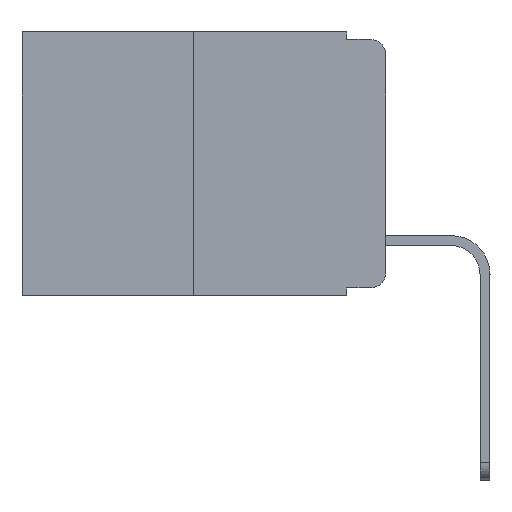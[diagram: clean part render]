
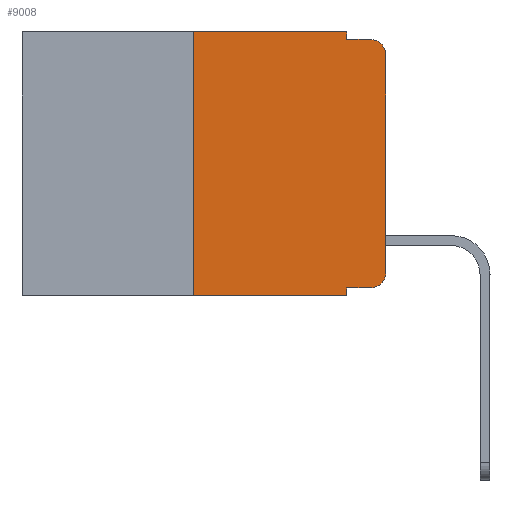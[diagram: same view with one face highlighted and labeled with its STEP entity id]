
A CAD part, left-side view. The second image highlights one B-rep face of the part: STEP entity #9008.
In plain terms, the highlighted planar face has unit normal (-1, 0, 0).
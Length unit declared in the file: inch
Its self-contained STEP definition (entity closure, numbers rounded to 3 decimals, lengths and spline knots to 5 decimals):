
#223 = DIRECTION ( 'NONE',  ( 0., 0., -1. ) ) ;
#382 = VECTOR ( 'NONE', #21145, 39.37008 ) ;
#999 = ORIENTED_EDGE ( 'NONE', *, *, #10594, .T. ) ;
#1274 = ORIENTED_EDGE ( 'NONE', *, *, #8105, .F. ) ;
#1292 = CARTESIAN_POINT ( 'NONE',  ( 0., 0.051, -0.01 ) ) ;
#1571 = LINE ( 'NONE', #1292, #16243 ) ;
#1714 = AXIS2_PLACEMENT_3D ( 'NONE', #18914, #5463, #12888 ) ;
#1986 = LINE ( 'NONE', #21783, #19339 ) ;
#3263 = VECTOR ( 'NONE', #16675, 39.37008 ) ;
#3325 = EDGE_CURVE ( 'NONE', #24397, #5724, #24232, .T. ) ;
#3365 = VERTEX_POINT ( 'NONE', #3757 ) ;
#3374 = LINE ( 'NONE', #19865, #17999 ) ;
#3675 = CARTESIAN_POINT ( 'NONE',  ( 0., 0.02, -0.313 ) ) ;
#3757 = CARTESIAN_POINT ( 'NONE',  ( 0., 0.02, -0.333 ) ) ;
#3808 = AXIS2_PLACEMENT_3D ( 'NONE', #21748, #19590, #4453 ) ;
#4098 = CARTESIAN_POINT ( 'NONE',  ( 0., 0., -0.313 ) ) ;
#4406 = VERTEX_POINT ( 'NONE', #22919 ) ;
#4453 = DIRECTION ( 'NONE',  ( 0., 0., -1. ) ) ;
#4575 = CARTESIAN_POINT ( 'NONE',  ( 0., 0.051, -0.01 ) ) ;
#5459 = ORIENTED_EDGE ( 'NONE', *, *, #3325, .F. ) ;
#5463 = DIRECTION ( 'NONE',  ( 1., 0., 0. ) ) ;
#5475 = LINE ( 'NONE', #19209, #382 ) ;
#5657 = LINE ( 'NONE', #22205, #3263 ) ;
#5724 = VERTEX_POINT ( 'NONE', #19797 ) ;
#6496 = CARTESIAN_POINT ( 'NONE',  ( 0., 0.02, -0.01 ) ) ;
#6886 = FACE_OUTER_BOUND ( 'NONE', #18349, .T. ) ;
#7477 = CARTESIAN_POINT ( 'NONE',  ( 0., 0.051, 0. ) ) ;
#7679 = DIRECTION ( 'NONE',  ( 0., -1., 0. ) ) ;
#7895 = DIRECTION ( 'NONE',  ( -1., 0., 0. ) ) ;
#8011 = EDGE_CURVE ( 'NONE', #3365, #12270, #15066, .T. ) ;
#8105 = EDGE_CURVE ( 'NONE', #4406, #22142, #5475, .T. ) ;
#8216 = EDGE_CURVE ( 'NONE', #22142, #20481, #3374, .T. ) ;
#8258 = VERTEX_POINT ( 'NONE', #21695 ) ;
#8381 = DIRECTION ( 'NONE',  ( 0., 0., 1. ) ) ;
#8938 = ORIENTED_EDGE ( 'NONE', *, *, #20327, .T. ) ;
#9008 = ADVANCED_FACE ( 'NONE', ( #6886 ), #16899, .F. ) ;
#9834 = VECTOR ( 'NONE', #7679, 39.37008 ) ;
#10045 = AXIS2_PLACEMENT_3D ( 'NONE', #3675, #7895, #223 ) ;
#10594 = EDGE_CURVE ( 'NONE', #8258, #21577, #18834, .T. ) ;
#10911 = ORIENTED_EDGE ( 'NONE', *, *, #8011, .T. ) ;
#11702 = LINE ( 'NONE', #23526, #12006 ) ;
#11826 = DIRECTION ( 'NONE',  ( 0., -1., 0. ) ) ;
#11882 = ORIENTED_EDGE ( 'NONE', *, *, #22261, .F. ) ;
#12006 = VECTOR ( 'NONE', #11826, 39.37008 ) ;
#12270 = VERTEX_POINT ( 'NONE', #4098 ) ;
#12397 = ORIENTED_EDGE ( 'NONE', *, *, #8216, .F. ) ;
#12503 = VERTEX_POINT ( 'NONE', #18258 ) ;
#12888 = DIRECTION ( 'NONE',  ( 0., 0., -1. ) ) ;
#13423 = EDGE_CURVE ( 'NONE', #24397, #3365, #23031, .T. ) ;
#13765 = CARTESIAN_POINT ( 'NONE',  ( 0., 0.051, 0. ) ) ;
#14480 = EDGE_CURVE ( 'NONE', #12503, #4406, #5657, .T. ) ;
#15066 = CIRCLE ( 'NONE', #10045, 0.02 ) ;
#15918 = ORIENTED_EDGE ( 'NONE', *, *, #14480, .F. ) ;
#16243 = VECTOR ( 'NONE', #24058, 39.37008 ) ;
#16675 = DIRECTION ( 'NONE',  ( 0., 0., 1. ) ) ;
#16899 = PLANE ( 'NONE',  #1714 ) ;
#17999 = VECTOR ( 'NONE', #21773, 39.37008 ) ;
#18258 = CARTESIAN_POINT ( 'NONE',  ( 0., 0.25, -0.343 ) ) ;
#18349 = EDGE_LOOP ( 'NONE', ( #8938, #999, #11882, #12397, #1274, #15918, #20696, #5459, #20070, #10911 ) ) ;
#18460 = EDGE_CURVE ( 'NONE', #12503, #5724, #11702, .T. ) ;
#18834 = CIRCLE ( 'NONE', #3808, 0.02 ) ;
#18914 = CARTESIAN_POINT ( 'NONE',  ( 0., 0.473, 0. ) ) ;
#19209 = CARTESIAN_POINT ( 'NONE',  ( 0., 0.473, 0. ) ) ;
#19339 = VECTOR ( 'NONE', #8381, 39.37008 ) ;
#19590 = DIRECTION ( 'NONE',  ( -1., 0., 0. ) ) ;
#19797 = CARTESIAN_POINT ( 'NONE',  ( 0., 0.051, -0.343 ) ) ;
#19865 = CARTESIAN_POINT ( 'NONE',  ( 0., 0.051, 0. ) ) ;
#20070 = ORIENTED_EDGE ( 'NONE', *, *, #13423, .T. ) ;
#20206 = CARTESIAN_POINT ( 'NONE',  ( 0., 0.051, -0.333 ) ) ;
#20327 = EDGE_CURVE ( 'NONE', #12270, #8258, #1986, .T. ) ;
#20344 = VECTOR ( 'NONE', #22579, 39.37008 ) ;
#20481 = VERTEX_POINT ( 'NONE', #4575 ) ;
#20696 = ORIENTED_EDGE ( 'NONE', *, *, #18460, .T. ) ;
#21145 = DIRECTION ( 'NONE',  ( 0., -1., 0. ) ) ;
#21577 = VERTEX_POINT ( 'NONE', #6496 ) ;
#21695 = CARTESIAN_POINT ( 'NONE',  ( 0., 0., -0.03 ) ) ;
#21748 = CARTESIAN_POINT ( 'NONE',  ( 0., 0.02, -0.03 ) ) ;
#21773 = DIRECTION ( 'NONE',  ( 0., 0., -1. ) ) ;
#21783 = CARTESIAN_POINT ( 'NONE',  ( 0., 0., 0. ) ) ;
#22142 = VERTEX_POINT ( 'NONE', #13765 ) ;
#22205 = CARTESIAN_POINT ( 'NONE',  ( 0., 0.25, 0. ) ) ;
#22261 = EDGE_CURVE ( 'NONE', #20481, #21577, #1571, .T. ) ;
#22579 = DIRECTION ( 'NONE',  ( 0., 0., -1. ) ) ;
#22919 = CARTESIAN_POINT ( 'NONE',  ( 0., 0.25, 0. ) ) ;
#23031 = LINE ( 'NONE', #23261, #9834 ) ;
#23261 = CARTESIAN_POINT ( 'NONE',  ( 0., 0.051, -0.333 ) ) ;
#23526 = CARTESIAN_POINT ( 'NONE',  ( 0., 0.473, -0.343 ) ) ;
#24058 = DIRECTION ( 'NONE',  ( 0., -1., 0. ) ) ;
#24232 = LINE ( 'NONE', #7477, #20344 ) ;
#24397 = VERTEX_POINT ( 'NONE', #20206 ) ;
